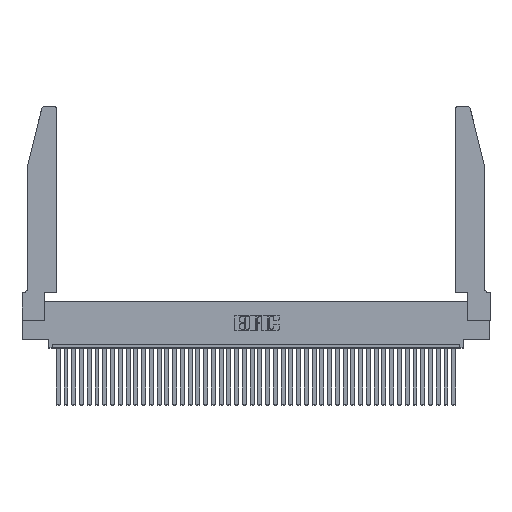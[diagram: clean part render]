
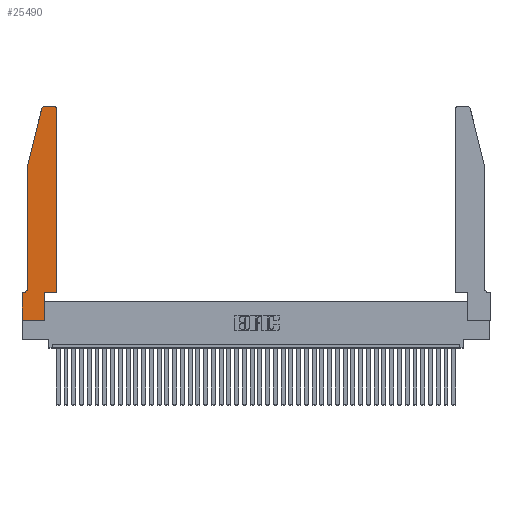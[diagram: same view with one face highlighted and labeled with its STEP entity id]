
A CAD part, top view. The second image highlights one B-rep face of the part: STEP entity #25490.
In plain terms, the highlighted planar face has unit normal (0, 0, 1).
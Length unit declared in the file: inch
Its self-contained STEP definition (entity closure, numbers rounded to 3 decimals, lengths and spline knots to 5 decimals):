
#34 = DIRECTION ( 'NONE',  ( 1., 0., 0. ) ) ;
#315 = CARTESIAN_POINT ( 'NONE',  ( 0.0755, 2., 0.37 ) ) ;
#447 = ORIENTED_EDGE ( 'NONE', *, *, #11534, .T. ) ;
#882 = DIRECTION ( 'NONE',  ( -0.239, -0.971, 0. ) ) ;
#1103 = CARTESIAN_POINT ( 'NONE',  ( 0., 0., 0.37 ) ) ;
#1444 = CARTESIAN_POINT ( 'NONE',  ( 0.0755, 2., 0.37 ) ) ;
#1541 = DIRECTION ( 'NONE',  ( 0., 0., -1. ) ) ;
#2424 = EDGE_CURVE ( 'NONE', #19866, #3016, #12159, .T. ) ;
#2672 = LINE ( 'NONE', #20441, #26304 ) ;
#2979 = EDGE_CURVE ( 'NONE', #21490, #18219, #37794, .T. ) ;
#3016 = VERTEX_POINT ( 'NONE', #36428 ) ;
#3475 = VECTOR ( 'NONE', #39164, 39.37008 ) ;
#3479 = CARTESIAN_POINT ( 'NONE',  ( 0.0755, 0.42, 0.37 ) ) ;
#4492 = ORIENTED_EDGE ( 'NONE', *, *, #2979, .T. ) ;
#4793 = AXIS2_PLACEMENT_3D ( 'NONE', #9739, #39342, #34 ) ;
#5036 = CARTESIAN_POINT ( 'NONE',  ( 0.4505, 2.72, 0.37 ) ) ;
#5043 = DIRECTION ( 'NONE',  ( -1., 0., 0. ) ) ;
#5390 = VECTOR ( 'NONE', #31902, 39.37008 ) ;
#5408 = ORIENTED_EDGE ( 'NONE', *, *, #2424, .T. ) ;
#6300 = EDGE_CURVE ( 'NONE', #31617, #42225, #6579, .T. ) ;
#6579 = LINE ( 'NONE', #7094, #14205 ) ;
#6820 = CARTESIAN_POINT ( 'NONE',  ( 0.0755, 2., 0.37 ) ) ;
#7094 = CARTESIAN_POINT ( 'NONE',  ( 0.0755, 0.35, 0.37 ) ) ;
#8943 = ORIENTED_EDGE ( 'NONE', *, *, #35425, .T. ) ;
#8948 = CARTESIAN_POINT ( 'NONE',  ( 0.2605, 2.75, 0.37 ) ) ;
#9393 = LINE ( 'NONE', #1444, #33995 ) ;
#9617 = AXIS2_PLACEMENT_3D ( 'NONE', #25282, #19770, #32703 ) ;
#9739 = CARTESIAN_POINT ( 'NONE',  ( 0.284, 2.72, 0.37 ) ) ;
#9889 = LINE ( 'NONE', #315, #12948 ) ;
#10008 = VERTEX_POINT ( 'NONE', #21066 ) ;
#10872 = DIRECTION ( 'NONE',  ( 0., -1., 0. ) ) ;
#11534 = EDGE_CURVE ( 'NONE', #21055, #40647, #9889, .T. ) ;
#11728 = ORIENTED_EDGE ( 'NONE', *, *, #21102, .T. ) ;
#12159 = LINE ( 'NONE', #32111, #3475 ) ;
#12417 = AXIS2_PLACEMENT_3D ( 'NONE', #14575, #1541, #5043 ) ;
#12948 = VECTOR ( 'NONE', #10872, 39.37008 ) ;
#13000 = VERTEX_POINT ( 'NONE', #5036 ) ;
#13268 = CARTESIAN_POINT ( 'NONE',  ( 0., 0., 0.37 ) ) ;
#13519 = DIRECTION ( 'NONE',  ( 0., 0., 1. ) ) ;
#13630 = ORIENTED_EDGE ( 'NONE', *, *, #34180, .T. ) ;
#14001 = VECTOR ( 'NONE', #18095, 39.37008 ) ;
#14205 = VECTOR ( 'NONE', #14503, 39.37008 ) ;
#14503 = DIRECTION ( 'NONE',  ( -1., 0., 0. ) ) ;
#14575 = CARTESIAN_POINT ( 'NONE',  ( 0.0055, 0.42, 0.37 ) ) ;
#14625 = AXIS2_PLACEMENT_3D ( 'NONE', #16816, #13519, #30040 ) ;
#15183 = ORIENTED_EDGE ( 'NONE', *, *, #23198, .T. ) ;
#15313 = VECTOR ( 'NONE', #24322, 39.37008 ) ;
#15555 = LINE ( 'NONE', #17517, #14001 ) ;
#15768 = CIRCLE ( 'NONE', #12417, 0.07 ) ;
#16816 = CARTESIAN_POINT ( 'NONE',  ( 0.4205, 2.72, 0.37 ) ) ;
#17517 = CARTESIAN_POINT ( 'NONE',  ( 0.4505, 0.35, 0.37 ) ) ;
#17760 = ORIENTED_EDGE ( 'NONE', *, *, #26625, .T. ) ;
#18095 = DIRECTION ( 'NONE',  ( 0., 1., 0. ) ) ;
#18219 = VERTEX_POINT ( 'NONE', #40477 ) ;
#19770 = DIRECTION ( 'NONE',  ( 0., 0., 1. ) ) ;
#19866 = VERTEX_POINT ( 'NONE', #21694 ) ;
#20441 = CARTESIAN_POINT ( 'NONE',  ( 0.4505, 0.35, 0.37 ) ) ;
#21055 = VERTEX_POINT ( 'NONE', #6820 ) ;
#21066 = CARTESIAN_POINT ( 'NONE',  ( 0.4205, 2.75, 0.37 ) ) ;
#21102 = EDGE_CURVE ( 'NONE', #27900, #19866, #38854, .T. ) ;
#21490 = VERTEX_POINT ( 'NONE', #34972 ) ;
#21694 = CARTESIAN_POINT ( 'NONE',  ( 0.2865, 0., 0.37 ) ) ;
#21861 = CARTESIAN_POINT ( 'NONE',  ( 0., 0.35, 0.37 ) ) ;
#22384 = PLANE ( 'NONE',  #9617 ) ;
#22780 = LINE ( 'NONE', #8948, #5390 ) ;
#23198 = EDGE_CURVE ( 'NONE', #28801, #13000, #15555, .T. ) ;
#23296 = EDGE_CURVE ( 'NONE', #10008, #21490, #22780, .T. ) ;
#23411 = EDGE_CURVE ( 'NONE', #18219, #21055, #9393, .T. ) ;
#24322 = DIRECTION ( 'NONE',  ( 0., -1., 0. ) ) ;
#24469 = CIRCLE ( 'NONE', #14625, 0.03 ) ;
#25282 = CARTESIAN_POINT ( 'NONE',  ( 0., 0.35, 0.37 ) ) ;
#25490 = ADVANCED_FACE ( 'NONE', ( #35359 ), #22384, .T. ) ;
#26304 = VECTOR ( 'NONE', #40283, 39.37008 ) ;
#26605 = EDGE_LOOP ( 'NONE', ( #33742, #4492, #34274, #447, #27889, #30578, #13630, #11728, #5408, #17760, #15183, #8943 ) ) ;
#26625 = EDGE_CURVE ( 'NONE', #3016, #28801, #2672, .T. ) ;
#27288 = CARTESIAN_POINT ( 'NONE',  ( 0., 0., 0.37 ) ) ;
#27889 = ORIENTED_EDGE ( 'NONE', *, *, #34970, .T. ) ;
#27900 = VERTEX_POINT ( 'NONE', #13268 ) ;
#28675 = LINE ( 'NONE', #1103, #15313 ) ;
#28801 = VERTEX_POINT ( 'NONE', #36711 ) ;
#30040 = DIRECTION ( 'NONE',  ( 1., 0., 0. ) ) ;
#30088 = VECTOR ( 'NONE', #34013, 39.37008 ) ;
#30578 = ORIENTED_EDGE ( 'NONE', *, *, #6300, .T. ) ;
#31617 = VERTEX_POINT ( 'NONE', #37004 ) ;
#31902 = DIRECTION ( 'NONE',  ( -1., 0., 0. ) ) ;
#32111 = CARTESIAN_POINT ( 'NONE',  ( 0.2865, 0.35, 0.37 ) ) ;
#32703 = DIRECTION ( 'NONE',  ( 1., 0., 0. ) ) ;
#33742 = ORIENTED_EDGE ( 'NONE', *, *, #23296, .T. ) ;
#33995 = VECTOR ( 'NONE', #882, 39.37008 ) ;
#34013 = DIRECTION ( 'NONE',  ( 1., 0., 0. ) ) ;
#34180 = EDGE_CURVE ( 'NONE', #42225, #27900, #28675, .T. ) ;
#34274 = ORIENTED_EDGE ( 'NONE', *, *, #23411, .T. ) ;
#34970 = EDGE_CURVE ( 'NONE', #40647, #31617, #15768, .T. ) ;
#34972 = CARTESIAN_POINT ( 'NONE',  ( 0.284, 2.75, 0.37 ) ) ;
#35359 = FACE_OUTER_BOUND ( 'NONE', #26605, .T. ) ;
#35425 = EDGE_CURVE ( 'NONE', #13000, #10008, #24469, .T. ) ;
#36428 = CARTESIAN_POINT ( 'NONE',  ( 0.2865, 0.35, 0.37 ) ) ;
#36711 = CARTESIAN_POINT ( 'NONE',  ( 0.4505, 0.35, 0.37 ) ) ;
#37004 = CARTESIAN_POINT ( 'NONE',  ( 0.0055, 0.35, 0.37 ) ) ;
#37794 = CIRCLE ( 'NONE', #4793, 0.03 ) ;
#38854 = LINE ( 'NONE', #27288, #30088 ) ;
#39164 = DIRECTION ( 'NONE',  ( 0., 1., 0. ) ) ;
#39342 = DIRECTION ( 'NONE',  ( 0., 0., 1. ) ) ;
#40283 = DIRECTION ( 'NONE',  ( 1., 0., 0. ) ) ;
#40477 = CARTESIAN_POINT ( 'NONE',  ( 0.25487, 2.72718, 0.37 ) ) ;
#40647 = VERTEX_POINT ( 'NONE', #3479 ) ;
#42225 = VERTEX_POINT ( 'NONE', #21861 ) ;
